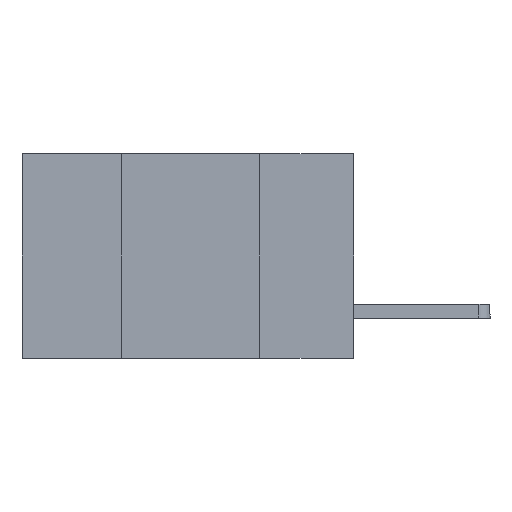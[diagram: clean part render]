
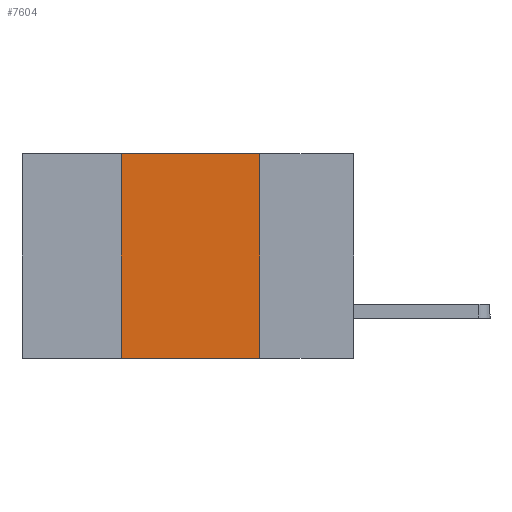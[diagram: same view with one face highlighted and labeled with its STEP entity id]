
A CAD part, left-side view. The second image highlights one B-rep face of the part: STEP entity #7604.
In plain terms, the highlighted planar face has unit normal (-1, 0, 0).
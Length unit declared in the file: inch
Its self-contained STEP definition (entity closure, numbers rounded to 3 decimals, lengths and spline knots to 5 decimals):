
#349 = DIRECTION ( 'NONE',  ( 0., -1., 0. ) ) ;
#443 = VERTEX_POINT ( 'NONE', #788 ) ;
#548 = CARTESIAN_POINT ( 'NONE',  ( 0., 0.6, -0.37 ) ) ;
#560 = EDGE_CURVE ( 'NONE', #666, #7170, #6391, .T. ) ;
#666 = VERTEX_POINT ( 'NONE', #4608 ) ;
#788 = CARTESIAN_POINT ( 'NONE',  ( 0., 0.42, -0.37 ) ) ;
#794 = VERTEX_POINT ( 'NONE', #7259 ) ;
#928 = VECTOR ( 'NONE', #2831, 39.37008 ) ;
#1700 = EDGE_CURVE ( 'NONE', #7170, #794, #1981, .T. ) ;
#1981 = LINE ( 'NONE', #5376, #5901 ) ;
#1988 = CARTESIAN_POINT ( 'NONE',  ( 0., 0.42, 0. ) ) ;
#2289 = VECTOR ( 'NONE', #6213, 39.37008 ) ;
#2831 = DIRECTION ( 'NONE',  ( 0., 0., 1. ) ) ;
#2928 = DIRECTION ( 'NONE',  ( 0., 0., -1. ) ) ;
#3456 = PLANE ( 'NONE',  #4331 ) ;
#4247 = EDGE_CURVE ( 'NONE', #443, #794, #6231, .T. ) ;
#4255 = VECTOR ( 'NONE', #349, 39.37008 ) ;
#4271 = DIRECTION ( 'NONE',  ( 1., 0., 0. ) ) ;
#4331 = AXIS2_PLACEMENT_3D ( 'NONE', #7950, #4271, #9382 ) ;
#4416 = CARTESIAN_POINT ( 'NONE',  ( 0., 0.6, 0. ) ) ;
#4608 = CARTESIAN_POINT ( 'NONE',  ( 0., 0.42, 0. ) ) ;
#4627 = ORIENTED_EDGE ( 'NONE', *, *, #560, .F. ) ;
#4672 = CARTESIAN_POINT ( 'NONE',  ( 0., 0.17, 0. ) ) ;
#5376 = CARTESIAN_POINT ( 'NONE',  ( 0., 0.17, 0. ) ) ;
#5901 = VECTOR ( 'NONE', #2928, 39.37008 ) ;
#6026 = FACE_OUTER_BOUND ( 'NONE', #8920, .T. ) ;
#6084 = ORIENTED_EDGE ( 'NONE', *, *, #1700, .F. ) ;
#6213 = DIRECTION ( 'NONE',  ( 0., -1., 0. ) ) ;
#6231 = LINE ( 'NONE', #548, #4255 ) ;
#6391 = LINE ( 'NONE', #4416, #2289 ) ;
#6990 = EDGE_CURVE ( 'NONE', #443, #666, #7235, .T. ) ;
#7048 = ORIENTED_EDGE ( 'NONE', *, *, #6990, .F. ) ;
#7170 = VERTEX_POINT ( 'NONE', #4672 ) ;
#7235 = LINE ( 'NONE', #1988, #928 ) ;
#7259 = CARTESIAN_POINT ( 'NONE',  ( 0., 0.17, -0.37 ) ) ;
#7374 = ORIENTED_EDGE ( 'NONE', *, *, #4247, .T. ) ;
#7604 = ADVANCED_FACE ( 'NONE', ( #6026 ), #3456, .F. ) ;
#7950 = CARTESIAN_POINT ( 'NONE',  ( 0., 0.6, 0. ) ) ;
#8920 = EDGE_LOOP ( 'NONE', ( #6084, #4627, #7048, #7374 ) ) ;
#9382 = DIRECTION ( 'NONE',  ( 0., 0., -1. ) ) ;
